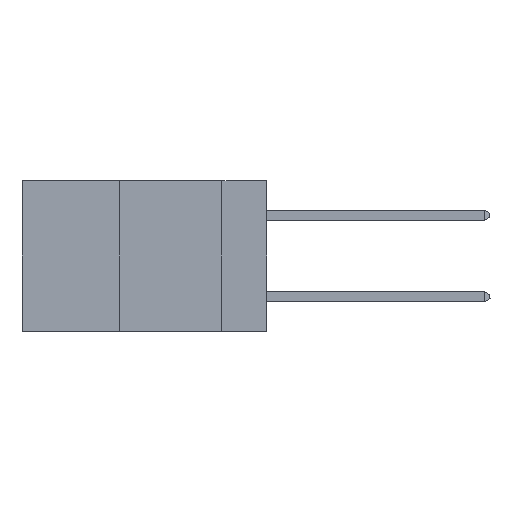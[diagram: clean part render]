
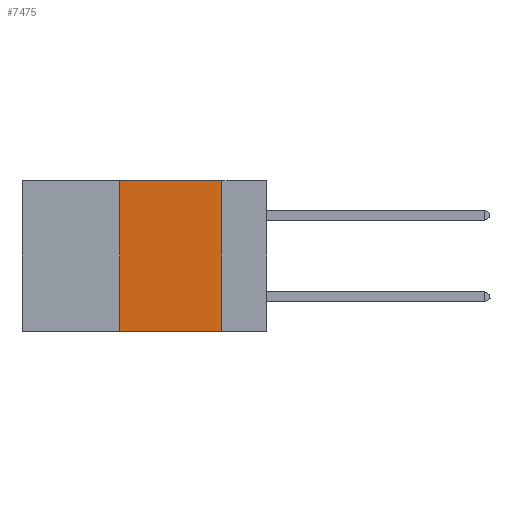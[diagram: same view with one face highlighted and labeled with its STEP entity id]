
A CAD part, left-side view. The second image highlights one B-rep face of the part: STEP entity #7475.
In plain terms, the highlighted planar face has unit normal (-1, 0, 0).
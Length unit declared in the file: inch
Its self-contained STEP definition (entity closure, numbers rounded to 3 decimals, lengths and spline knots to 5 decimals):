
#28 = CARTESIAN_POINT ( 'NONE',  ( 0., 0.6, 0. ) ) ;
#123 = CARTESIAN_POINT ( 'NONE',  ( 0., 0.36, 0. ) ) ;
#415 = CARTESIAN_POINT ( 'NONE',  ( 0., 0.6, -0.37 ) ) ;
#1192 = LINE ( 'NONE', #11108, #6482 ) ;
#1361 = VERTEX_POINT ( 'NONE', #7399 ) ;
#1802 = FACE_OUTER_BOUND ( 'NONE', #3054, .T. ) ;
#1906 = CARTESIAN_POINT ( 'NONE',  ( 0., 0.36, 0. ) ) ;
#2689 = CARTESIAN_POINT ( 'NONE',  ( 0., 0.6, 0. ) ) ;
#3054 = EDGE_LOOP ( 'NONE', ( #20324, #17599, #11823, #10792 ) ) ;
#3693 = DIRECTION ( 'NONE',  ( 0., 0., 1. ) ) ;
#3766 = LINE ( 'NONE', #1906, #14754 ) ;
#4302 = DIRECTION ( 'NONE',  ( 0., 0., -1. ) ) ;
#4576 = VERTEX_POINT ( 'NONE', #8182 ) ;
#4969 = AXIS2_PLACEMENT_3D ( 'NONE', #2689, #13850, #4302 ) ;
#6482 = VECTOR ( 'NONE', #12493, 39.37008 ) ;
#7399 = CARTESIAN_POINT ( 'NONE',  ( 0., 0.11, -0.37 ) ) ;
#7475 = ADVANCED_FACE ( 'NONE', ( #1802 ), #17117, .F. ) ;
#8182 = CARTESIAN_POINT ( 'NONE',  ( 0., 0.36, -0.37 ) ) ;
#8564 = LINE ( 'NONE', #415, #17609 ) ;
#9049 = EDGE_CURVE ( 'NONE', #4576, #18721, #3766, .T. ) ;
#9437 = VECTOR ( 'NONE', #9961, 39.37008 ) ;
#9961 = DIRECTION ( 'NONE',  ( 0., -1., 0. ) ) ;
#10054 = EDGE_CURVE ( 'NONE', #20051, #1361, #1192, .T. ) ;
#10792 = ORIENTED_EDGE ( 'NONE', *, *, #16211, .T. ) ;
#11108 = CARTESIAN_POINT ( 'NONE',  ( 0., 0.11, 0. ) ) ;
#11285 = CARTESIAN_POINT ( 'NONE',  ( 0., 0.11, 0. ) ) ;
#11685 = DIRECTION ( 'NONE',  ( 0., -1., 0. ) ) ;
#11823 = ORIENTED_EDGE ( 'NONE', *, *, #9049, .F. ) ;
#12493 = DIRECTION ( 'NONE',  ( 0., 0., -1. ) ) ;
#12915 = EDGE_CURVE ( 'NONE', #18721, #20051, #14174, .T. ) ;
#13850 = DIRECTION ( 'NONE',  ( 1., 0., 0. ) ) ;
#14174 = LINE ( 'NONE', #28, #9437 ) ;
#14754 = VECTOR ( 'NONE', #3693, 39.37008 ) ;
#16211 = EDGE_CURVE ( 'NONE', #4576, #1361, #8564, .T. ) ;
#17117 = PLANE ( 'NONE',  #4969 ) ;
#17599 = ORIENTED_EDGE ( 'NONE', *, *, #12915, .F. ) ;
#17609 = VECTOR ( 'NONE', #11685, 39.37008 ) ;
#18721 = VERTEX_POINT ( 'NONE', #123 ) ;
#20051 = VERTEX_POINT ( 'NONE', #11285 ) ;
#20324 = ORIENTED_EDGE ( 'NONE', *, *, #10054, .F. ) ;
